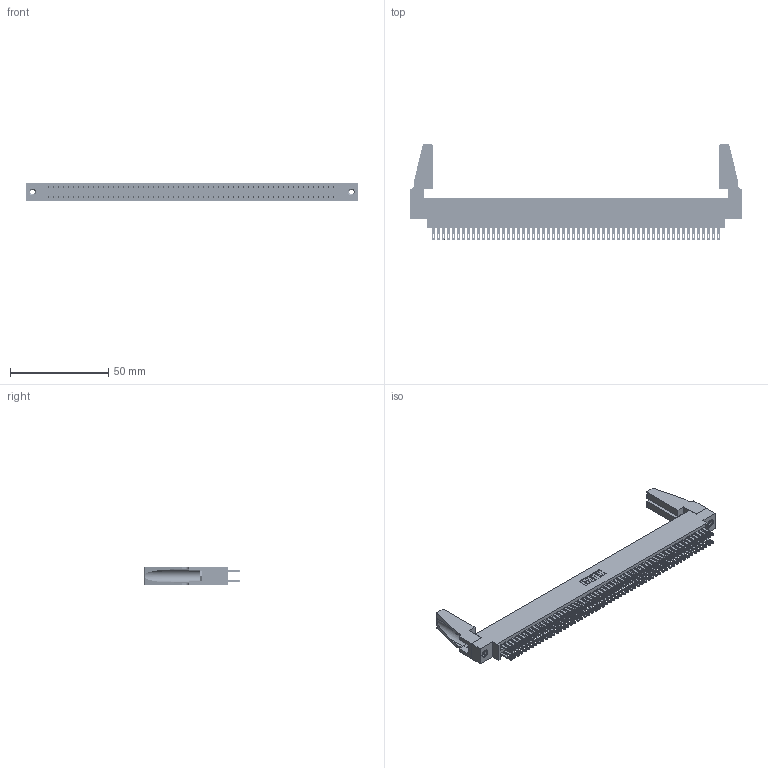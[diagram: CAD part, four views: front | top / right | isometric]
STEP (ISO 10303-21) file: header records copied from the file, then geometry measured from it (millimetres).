
FILE_DESCRIPTION (( 'STEP AP203' ), '1' );
FILE_NAME ('345-116-500-888.STEP', '2019-11-05T13:47:28', ( '' ), ( '' ), 'SwSTEP 2.0', 'SolidWorks 2016', '' );
FILE_SCHEMA (( 'CONFIG_CONTROL_DESIGN' ));
Length unit declared in the file: inch
Products named in the file (5): 345-116-500-888; 345-220-078_345-220-088; 345 Part_0.170 Offset - 0.156 Dia-TH; 345-250-001_345-250-001-102; 345-292-001_345-293-100
Assembly tree (121 placements, depth 2):
  345-116-500-888
    345 Part_0.170 Offset - 0.156 Dia-TH
    345-292-001_345-293-100  x116
    345-250-001_345-250-001-102  x2
    345-220-078_345-220-088  x2
Bounding box: 168.55 x 48.69 x 9.4 mm (x, y, z)
Volume: 20015.6 mm3; surface area: 29537.4 mm2
Topology: 121 solids, 121 shells, 5590 faces, 17023 edges, 11338 vertices
Faces by surface type: plane 3288, cylinder 2286, cone 12, torus 4
Entity records: 45564 total; most frequent: CARTESIAN_POINT 7618, ORIENTED_EDGE 7512, DIRECTION 6704, EDGE_CURVE 3756, LINE 3346, VECTOR 3346, VERTEX_POINT 2498, AXIS2_PLACEMENT_3D 1679
